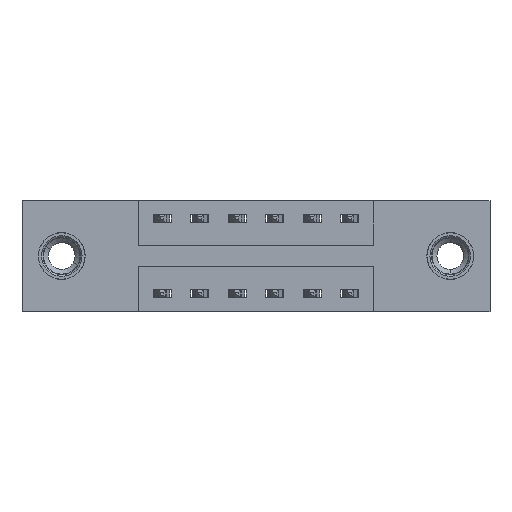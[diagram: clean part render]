
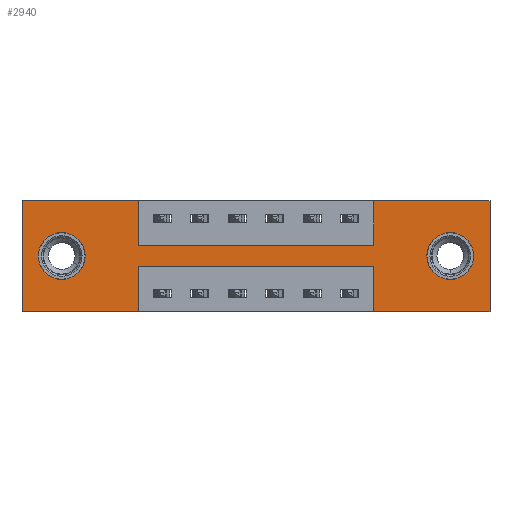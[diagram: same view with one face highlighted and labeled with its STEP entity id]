
A CAD part, front view. The second image highlights one B-rep face of the part: STEP entity #2940.
In plain terms, the highlighted planar face has unit normal (0, -1, 0).
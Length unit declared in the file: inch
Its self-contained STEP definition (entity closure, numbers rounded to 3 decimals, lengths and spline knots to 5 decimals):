
#6 = CARTESIAN_POINT ( 'NONE',  ( 1.1725, 0., 0. ) ) ;
#128 = CARTESIAN_POINT ( 'NONE',  ( 1.1725, 0., -0.22 ) ) ;
#341 = VERTEX_POINT ( 'NONE', #7603 ) ;
#501 = CIRCLE ( 'NONE', #4859, 0.078 ) ;
#727 = EDGE_CURVE ( 'NONE', #3247, #4049, #1018, .T. ) ;
#744 = CARTESIAN_POINT ( 'NONE',  ( 1.4275, 0., -0.185 ) ) ;
#745 = VECTOR ( 'NONE', #3566, 39.37008 ) ;
#922 = ORIENTED_EDGE ( 'NONE', *, *, #9331, .F. ) ;
#951 = CARTESIAN_POINT ( 'NONE',  ( 0., 0., 0. ) ) ;
#1018 = CIRCLE ( 'NONE', #9729, 0.078 ) ;
#1103 = AXIS2_PLACEMENT_3D ( 'NONE', #7191, #2546, #3224 ) ;
#1125 = DIRECTION ( 'NONE',  ( 0., 0., -1. ) ) ;
#1211 = EDGE_CURVE ( 'NONE', #7975, #6154, #4944, .T. ) ;
#1256 = VECTOR ( 'NONE', #6379, 39.37008 ) ;
#1337 = EDGE_CURVE ( 'NONE', #3965, #2859, #7227, .T. ) ;
#1452 = DIRECTION ( 'NONE',  ( 0., 1., 0. ) ) ;
#1760 = EDGE_LOOP ( 'NONE', ( #6526, #2666 ) ) ;
#1783 = ORIENTED_EDGE ( 'NONE', *, *, #7301, .F. ) ;
#1808 = EDGE_CURVE ( 'NONE', #341, #8914, #3205, .T. ) ;
#2000 = VERTEX_POINT ( 'NONE', #7145 ) ;
#2218 = CARTESIAN_POINT ( 'NONE',  ( 1.4275, 0., -0.263 ) ) ;
#2272 = CIRCLE ( 'NONE', #1103, 0.078 ) ;
#2341 = LINE ( 'NONE', #4537, #3800 ) ;
#2367 = ORIENTED_EDGE ( 'NONE', *, *, #1808, .F. ) ;
#2477 = VECTOR ( 'NONE', #6810, 39.37008 ) ;
#2478 = DIRECTION ( 'NONE',  ( 0., 0., 1. ) ) ;
#2542 = VERTEX_POINT ( 'NONE', #9736 ) ;
#2546 = DIRECTION ( 'NONE',  ( 0., 1., 0. ) ) ;
#2628 = VERTEX_POINT ( 'NONE', #2218 ) ;
#2666 = ORIENTED_EDGE ( 'NONE', *, *, #6869, .T. ) ;
#2670 = VECTOR ( 'NONE', #1125, 39.37008 ) ;
#2698 = ORIENTED_EDGE ( 'NONE', *, *, #3557, .F. ) ;
#2737 = EDGE_LOOP ( 'NONE', ( #1783, #922, #2367, #3003, #4454, #6173, #5799, #7085, #4710, #8074, #2698, #3197 ) ) ;
#2739 = CARTESIAN_POINT ( 'NONE',  ( 1.56, 0., 0. ) ) ;
#2765 = VERTEX_POINT ( 'NONE', #7865 ) ;
#2839 = PLANE ( 'NONE',  #6188 ) ;
#2859 = VERTEX_POINT ( 'NONE', #8086 ) ;
#2884 = AXIS2_PLACEMENT_3D ( 'NONE', #744, #3683, #6065 ) ;
#2911 = CARTESIAN_POINT ( 'NONE',  ( 0.1325, 0., -0.263 ) ) ;
#2940 = ADVANCED_FACE ( 'NONE', ( #4791, #4045, #8592 ), #2839, .T. ) ;
#2964 = CARTESIAN_POINT ( 'NONE',  ( 0.1325, 0., -0.185 ) ) ;
#3000 = EDGE_LOOP ( 'NONE', ( #6561, #9898 ) ) ;
#3003 = ORIENTED_EDGE ( 'NONE', *, *, #3272, .F. ) ;
#3036 = VECTOR ( 'NONE', #5721, 39.37008 ) ;
#3086 = CARTESIAN_POINT ( 'NONE',  ( 0., 0., -0.37 ) ) ;
#3197 = ORIENTED_EDGE ( 'NONE', *, *, #6425, .F. ) ;
#3205 = LINE ( 'NONE', #5429, #9103 ) ;
#3224 = DIRECTION ( 'NONE',  ( 0., 0., -1. ) ) ;
#3247 = VERTEX_POINT ( 'NONE', #5249 ) ;
#3272 = EDGE_CURVE ( 'NONE', #8050, #341, #2341, .T. ) ;
#3292 = EDGE_CURVE ( 'NONE', #2542, #5840, #9671, .T. ) ;
#3557 = EDGE_CURVE ( 'NONE', #2000, #2542, #3916, .T. ) ;
#3565 = LINE ( 'NONE', #9351, #6967 ) ;
#3566 = DIRECTION ( 'NONE',  ( 0., 0., 1. ) ) ;
#3682 = DIRECTION ( 'NONE',  ( 0., 0., -1. ) ) ;
#3683 = DIRECTION ( 'NONE',  ( 0., 1., 0. ) ) ;
#3792 = CARTESIAN_POINT ( 'NONE',  ( 0.3875, 0., -0.22 ) ) ;
#3800 = VECTOR ( 'NONE', #6844, 39.37008 ) ;
#3916 = LINE ( 'NONE', #8135, #745 ) ;
#3965 = VERTEX_POINT ( 'NONE', #5929 ) ;
#4045 = FACE_BOUND ( 'NONE', #3000, .T. ) ;
#4049 = VERTEX_POINT ( 'NONE', #2911 ) ;
#4454 = ORIENTED_EDGE ( 'NONE', *, *, #9178, .F. ) ;
#4537 = CARTESIAN_POINT ( 'NONE',  ( 0., 0., -0.37 ) ) ;
#4710 = ORIENTED_EDGE ( 'NONE', *, *, #9033, .F. ) ;
#4791 = FACE_BOUND ( 'NONE', #1760, .T. ) ;
#4859 = AXIS2_PLACEMENT_3D ( 'NONE', #9188, #1452, #2478 ) ;
#4944 = LINE ( 'NONE', #951, #1256 ) ;
#4962 = CARTESIAN_POINT ( 'NONE',  ( 0.3875, 0., -0.22 ) ) ;
#5081 = DIRECTION ( 'NONE',  ( 0., 0., -1. ) ) ;
#5202 = DIRECTION ( 'NONE',  ( 0., -1., 0. ) ) ;
#5249 = CARTESIAN_POINT ( 'NONE',  ( 0.1325, 0., -0.107 ) ) ;
#5279 = CARTESIAN_POINT ( 'NONE',  ( 0., 0., 0. ) ) ;
#5429 = CARTESIAN_POINT ( 'NONE',  ( 1.1725, 0., -0.37 ) ) ;
#5609 = VECTOR ( 'NONE', #7609, 39.37008 ) ;
#5717 = LINE ( 'NONE', #2739, #2670 ) ;
#5721 = DIRECTION ( 'NONE',  ( -1., 0., 0. ) ) ;
#5799 = ORIENTED_EDGE ( 'NONE', *, *, #9093, .F. ) ;
#5840 = VERTEX_POINT ( 'NONE', #6305 ) ;
#5929 = CARTESIAN_POINT ( 'NONE',  ( 0.3875, 0., -0.15 ) ) ;
#5956 = LINE ( 'NONE', #8072, #8099 ) ;
#6065 = DIRECTION ( 'NONE',  ( 0., 0., -1. ) ) ;
#6083 = DIRECTION ( 'NONE',  ( 0., 0., 1. ) ) ;
#6135 = VECTOR ( 'NONE', #8936, 39.37008 ) ;
#6154 = VERTEX_POINT ( 'NONE', #7330 ) ;
#6173 = ORIENTED_EDGE ( 'NONE', *, *, #1211, .F. ) ;
#6188 = AXIS2_PLACEMENT_3D ( 'NONE', #7591, #5202, #8209 ) ;
#6305 = CARTESIAN_POINT ( 'NONE',  ( 0.3875, 0., 0. ) ) ;
#6379 = DIRECTION ( 'NONE',  ( 1., 0., 0. ) ) ;
#6425 = EDGE_CURVE ( 'NONE', #2765, #2000, #7607, .T. ) ;
#6526 = ORIENTED_EDGE ( 'NONE', *, *, #6557, .T. ) ;
#6557 = EDGE_CURVE ( 'NONE', #9418, #2628, #8781, .T. ) ;
#6561 = ORIENTED_EDGE ( 'NONE', *, *, #727, .T. ) ;
#6648 = VECTOR ( 'NONE', #7874, 39.37008 ) ;
#6795 = DIRECTION ( 'NONE',  ( 0., 1., 0. ) ) ;
#6810 = DIRECTION ( 'NONE',  ( 1., 0., 0. ) ) ;
#6844 = DIRECTION ( 'NONE',  ( -1., 0., 0. ) ) ;
#6869 = EDGE_CURVE ( 'NONE', #2628, #9418, #2272, .T. ) ;
#6967 = VECTOR ( 'NONE', #3682, 39.37008 ) ;
#7085 = ORIENTED_EDGE ( 'NONE', *, *, #1337, .F. ) ;
#7145 = CARTESIAN_POINT ( 'NONE',  ( 0., 0., -0.37 ) ) ;
#7185 = CARTESIAN_POINT ( 'NONE',  ( 1.56, 0., -0.37 ) ) ;
#7191 = CARTESIAN_POINT ( 'NONE',  ( 1.4275, 0., -0.185 ) ) ;
#7227 = LINE ( 'NONE', #8836, #6135 ) ;
#7301 = EDGE_CURVE ( 'NONE', #9852, #2765, #3565, .T. ) ;
#7330 = CARTESIAN_POINT ( 'NONE',  ( 1.56, 0., 0. ) ) ;
#7591 = CARTESIAN_POINT ( 'NONE',  ( 0., 0., -0.37 ) ) ;
#7603 = CARTESIAN_POINT ( 'NONE',  ( 1.1725, 0., -0.37 ) ) ;
#7607 = LINE ( 'NONE', #3086, #6648 ) ;
#7609 = DIRECTION ( 'NONE',  ( 0., 0., 1. ) ) ;
#7740 = LINE ( 'NONE', #4962, #3036 ) ;
#7865 = CARTESIAN_POINT ( 'NONE',  ( 0.3875, 0., -0.37 ) ) ;
#7874 = DIRECTION ( 'NONE',  ( -1., 0., 0. ) ) ;
#7975 = VERTEX_POINT ( 'NONE', #8520 ) ;
#8050 = VERTEX_POINT ( 'NONE', #7185 ) ;
#8072 = CARTESIAN_POINT ( 'NONE',  ( 0.3875, 0., 0. ) ) ;
#8074 = ORIENTED_EDGE ( 'NONE', *, *, #3292, .F. ) ;
#8086 = CARTESIAN_POINT ( 'NONE',  ( 1.1725, 0., -0.15 ) ) ;
#8099 = VECTOR ( 'NONE', #5081, 39.37008 ) ;
#8135 = CARTESIAN_POINT ( 'NONE',  ( 0., 0., 0. ) ) ;
#8165 = EDGE_CURVE ( 'NONE', #4049, #3247, #501, .T. ) ;
#8209 = DIRECTION ( 'NONE',  ( 0., 0., -1. ) ) ;
#8446 = DIRECTION ( 'NONE',  ( 0., 0., 1. ) ) ;
#8520 = CARTESIAN_POINT ( 'NONE',  ( 1.1725, 0., 0. ) ) ;
#8592 = FACE_OUTER_BOUND ( 'NONE', #2737, .T. ) ;
#8781 = CIRCLE ( 'NONE', #2884, 0.078 ) ;
#8836 = CARTESIAN_POINT ( 'NONE',  ( 0.3875, 0., -0.15 ) ) ;
#8914 = VERTEX_POINT ( 'NONE', #128 ) ;
#8936 = DIRECTION ( 'NONE',  ( 1., 0., 0. ) ) ;
#9033 = EDGE_CURVE ( 'NONE', #5840, #3965, #5956, .T. ) ;
#9056 = CARTESIAN_POINT ( 'NONE',  ( 1.4275, 0., -0.107 ) ) ;
#9093 = EDGE_CURVE ( 'NONE', #2859, #7975, #9638, .T. ) ;
#9103 = VECTOR ( 'NONE', #8446, 39.37008 ) ;
#9178 = EDGE_CURVE ( 'NONE', #6154, #8050, #5717, .T. ) ;
#9188 = CARTESIAN_POINT ( 'NONE',  ( 0.1325, 0., -0.185 ) ) ;
#9331 = EDGE_CURVE ( 'NONE', #8914, #9852, #7740, .T. ) ;
#9351 = CARTESIAN_POINT ( 'NONE',  ( 0.3875, 0., -0.37 ) ) ;
#9418 = VERTEX_POINT ( 'NONE', #9056 ) ;
#9638 = LINE ( 'NONE', #6, #5609 ) ;
#9671 = LINE ( 'NONE', #5279, #2477 ) ;
#9729 = AXIS2_PLACEMENT_3D ( 'NONE', #2964, #6795, #6083 ) ;
#9736 = CARTESIAN_POINT ( 'NONE',  ( 0., 0., 0. ) ) ;
#9852 = VERTEX_POINT ( 'NONE', #3792 ) ;
#9898 = ORIENTED_EDGE ( 'NONE', *, *, #8165, .T. ) ;
